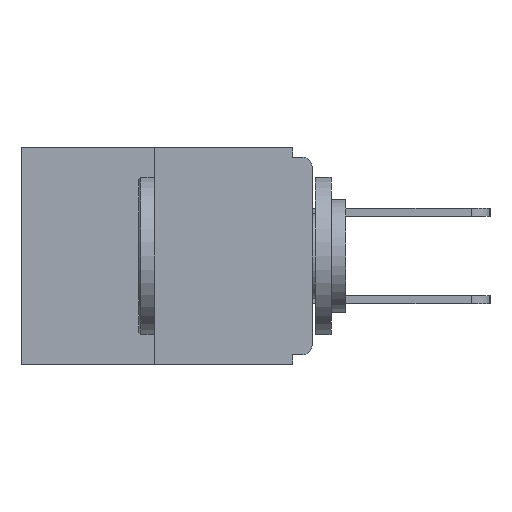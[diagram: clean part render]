
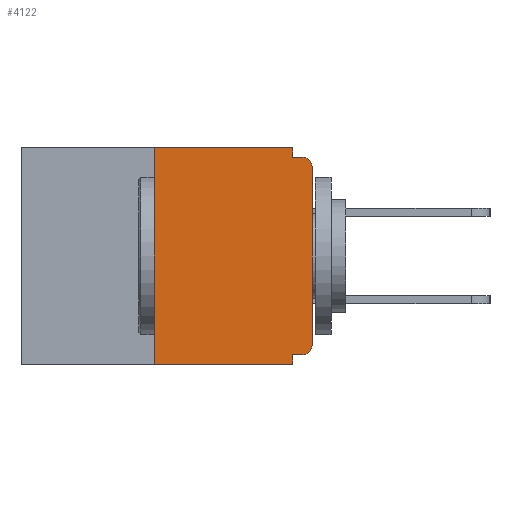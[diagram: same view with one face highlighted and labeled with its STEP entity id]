
A CAD part, left-side view. The second image highlights one B-rep face of the part: STEP entity #4122.
In plain terms, the highlighted planar face has unit normal (-1, 0, 0).
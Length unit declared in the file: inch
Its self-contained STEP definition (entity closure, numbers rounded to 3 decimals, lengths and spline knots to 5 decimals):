
#598 = ORIENTED_EDGE ( 'NONE', *, *, #13079, .T. ) ;
#599 = CARTESIAN_POINT ( 'NONE',  ( 0., 0., -0.313 ) ) ;
#1269 = CARTESIAN_POINT ( 'NONE',  ( 0., 0., -0.328 ) ) ;
#2099 = AXIS2_PLACEMENT_3D ( 'NONE', #28593, #21672, #28910 ) ;
#2142 = VERTEX_POINT ( 'NONE', #5333 ) ;
#2278 = CARTESIAN_POINT ( 'NONE',  ( 0., 0.031, 0. ) ) ;
#2339 = ORIENTED_EDGE ( 'NONE', *, *, #14212, .T. ) ;
#3196 = VECTOR ( 'NONE', #4545, 39.37008 ) ;
#3463 = CARTESIAN_POINT ( 'NONE',  ( 0., 0.015, -0.328 ) ) ;
#3632 = DIRECTION ( 'NONE',  ( 0., 1., 0. ) ) ;
#3716 = EDGE_CURVE ( 'NONE', #21442, #16545, #21087, .T. ) ;
#4021 = EDGE_CURVE ( 'NONE', #11050, #2142, #16677, .T. ) ;
#4122 = ADVANCED_FACE ( 'NONE', ( #22529 ), #24848, .F. ) ;
#4123 = DIRECTION ( 'NONE',  ( 1., 0., 0. ) ) ;
#4545 = DIRECTION ( 'NONE',  ( 0., -1., 0. ) ) ;
#4714 = ORIENTED_EDGE ( 'NONE', *, *, #29121, .F. ) ;
#4821 = ORIENTED_EDGE ( 'NONE', *, *, #14557, .F. ) ;
#5333 = CARTESIAN_POINT ( 'NONE',  ( 0., 0.031, -0.328 ) ) ;
#5998 = EDGE_LOOP ( 'NONE', ( #21427, #4821, #29589, #24654, #26170, #598, #28589, #2339, #7902, #4714 ) ) ;
#6276 = VERTEX_POINT ( 'NONE', #29970 ) ;
#6279 = VERTEX_POINT ( 'NONE', #15813 ) ;
#7266 = VERTEX_POINT ( 'NONE', #29707 ) ;
#7384 = EDGE_CURVE ( 'NONE', #7266, #10719, #20822, .T. ) ;
#7508 = CARTESIAN_POINT ( 'NONE',  ( 0., 0.031, -0.343 ) ) ;
#7521 = VECTOR ( 'NONE', #16988, 39.37008 ) ;
#7902 = ORIENTED_EDGE ( 'NONE', *, *, #7384, .F. ) ;
#9039 = VECTOR ( 'NONE', #26493, 39.37008 ) ;
#9112 = VECTOR ( 'NONE', #28769, 39.37008 ) ;
#10223 = VECTOR ( 'NONE', #13273, 39.37008 ) ;
#10719 = VERTEX_POINT ( 'NONE', #21982 ) ;
#11050 = VERTEX_POINT ( 'NONE', #3463 ) ;
#11254 = CARTESIAN_POINT ( 'NONE',  ( 0., 0., -0.015 ) ) ;
#11946 = CIRCLE ( 'NONE', #2099, 0.015 ) ;
#12632 = LINE ( 'NONE', #7508, #7521 ) ;
#13069 = LINE ( 'NONE', #28663, #9112 ) ;
#13079 = EDGE_CURVE ( 'NONE', #11050, #16713, #27304, .T. ) ;
#13184 = CARTESIAN_POINT ( 'NONE',  ( 0., 0., 0. ) ) ;
#13273 = DIRECTION ( 'NONE',  ( 0., 0., 1. ) ) ;
#13722 = CARTESIAN_POINT ( 'NONE',  ( 0., 0.46, 0. ) ) ;
#14212 = EDGE_CURVE ( 'NONE', #20072, #10719, #11946, .T. ) ;
#14557 = EDGE_CURVE ( 'NONE', #6276, #21442, #29430, .T. ) ;
#14608 = VECTOR ( 'NONE', #16260, 39.37008 ) ;
#15701 = LINE ( 'NONE', #13184, #10223 ) ;
#15764 = CARTESIAN_POINT ( 'NONE',  ( 0., 0.46, 0. ) ) ;
#15813 = CARTESIAN_POINT ( 'NONE',  ( 0., 0.031, -0.343 ) ) ;
#16260 = DIRECTION ( 'NONE',  ( 0., -1., 0. ) ) ;
#16490 = DIRECTION ( 'NONE',  ( -1., 0., 0. ) ) ;
#16545 = VERTEX_POINT ( 'NONE', #2278 ) ;
#16677 = LINE ( 'NONE', #1269, #18519 ) ;
#16713 = VERTEX_POINT ( 'NONE', #599 ) ;
#16988 = DIRECTION ( 'NONE',  ( 0., 0., -1. ) ) ;
#17237 = CARTESIAN_POINT ( 'NONE',  ( 0., 0., -0.03 ) ) ;
#18519 = VECTOR ( 'NONE', #3632, 39.37008 ) ;
#18790 = CARTESIAN_POINT ( 'NONE',  ( 0., 0.25, 0. ) ) ;
#19831 = AXIS2_PLACEMENT_3D ( 'NONE', #30118, #16490, #20962 ) ;
#19877 = AXIS2_PLACEMENT_3D ( 'NONE', #15764, #4123, #22826 ) ;
#20072 = VERTEX_POINT ( 'NONE', #17237 ) ;
#20822 = LINE ( 'NONE', #11254, #14608 ) ;
#20962 = DIRECTION ( 'NONE',  ( 0., 0., -1. ) ) ;
#21087 = LINE ( 'NONE', #13722, #3196 ) ;
#21427 = ORIENTED_EDGE ( 'NONE', *, *, #3716, .F. ) ;
#21442 = VERTEX_POINT ( 'NONE', #18790 ) ;
#21672 = DIRECTION ( 'NONE',  ( -1., 0., 0. ) ) ;
#21861 = DIRECTION ( 'NONE',  ( 0., 0., 1. ) ) ;
#21982 = CARTESIAN_POINT ( 'NONE',  ( 0., 0.015, -0.015 ) ) ;
#22529 = FACE_OUTER_BOUND ( 'NONE', #5998, .T. ) ;
#22727 = EDGE_CURVE ( 'NONE', #6276, #6279, #27269, .T. ) ;
#22826 = DIRECTION ( 'NONE',  ( 0., 0., -1. ) ) ;
#24003 = EDGE_CURVE ( 'NONE', #2142, #6279, #12632, .T. ) ;
#24654 = ORIENTED_EDGE ( 'NONE', *, *, #24003, .F. ) ;
#24848 = PLANE ( 'NONE',  #19877 ) ;
#26170 = ORIENTED_EDGE ( 'NONE', *, *, #4021, .F. ) ;
#26444 = CARTESIAN_POINT ( 'NONE',  ( 0., 0.25, 0. ) ) ;
#26493 = DIRECTION ( 'NONE',  ( 0., -1., 0. ) ) ;
#26785 = CARTESIAN_POINT ( 'NONE',  ( 0., 0.46, -0.343 ) ) ;
#27269 = LINE ( 'NONE', #26785, #9039 ) ;
#27304 = CIRCLE ( 'NONE', #19831, 0.015 ) ;
#27987 = VECTOR ( 'NONE', #21861, 39.37008 ) ;
#28589 = ORIENTED_EDGE ( 'NONE', *, *, #28661, .T. ) ;
#28593 = CARTESIAN_POINT ( 'NONE',  ( 0., 0.015, -0.03 ) ) ;
#28661 = EDGE_CURVE ( 'NONE', #16713, #20072, #15701, .T. ) ;
#28663 = CARTESIAN_POINT ( 'NONE',  ( 0., 0.031, 0. ) ) ;
#28769 = DIRECTION ( 'NONE',  ( 0., 0., -1. ) ) ;
#28910 = DIRECTION ( 'NONE',  ( 0., 0., -1. ) ) ;
#29121 = EDGE_CURVE ( 'NONE', #16545, #7266, #13069, .T. ) ;
#29430 = LINE ( 'NONE', #26444, #27987 ) ;
#29589 = ORIENTED_EDGE ( 'NONE', *, *, #22727, .T. ) ;
#29707 = CARTESIAN_POINT ( 'NONE',  ( 0., 0.031, -0.015 ) ) ;
#29970 = CARTESIAN_POINT ( 'NONE',  ( 0., 0.25, -0.343 ) ) ;
#30118 = CARTESIAN_POINT ( 'NONE',  ( 0., 0.015, -0.313 ) ) ;
